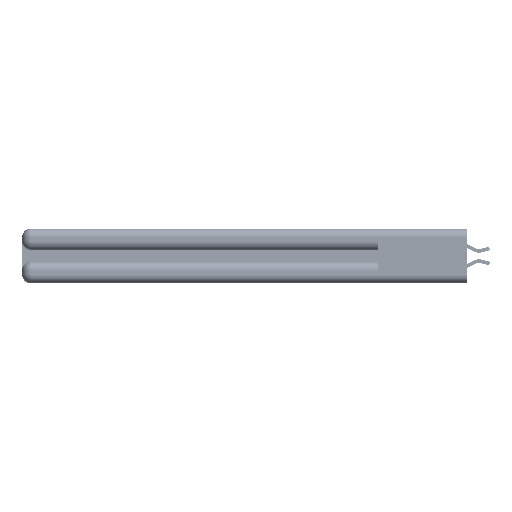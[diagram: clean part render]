
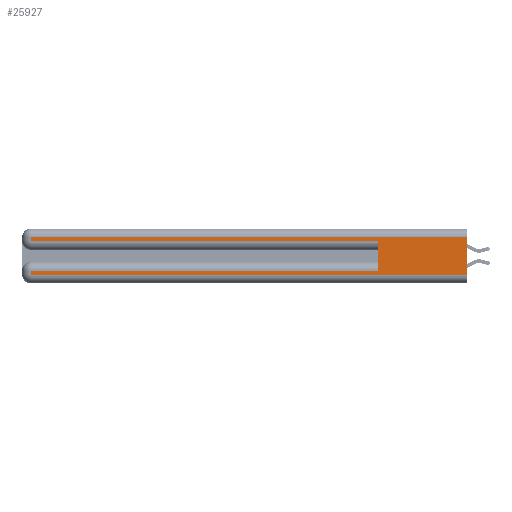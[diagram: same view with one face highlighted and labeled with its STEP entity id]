
A CAD part, left-side view. The second image highlights one B-rep face of the part: STEP entity #25927.
In plain terms, the highlighted planar face has unit normal (-1, 0, 0).
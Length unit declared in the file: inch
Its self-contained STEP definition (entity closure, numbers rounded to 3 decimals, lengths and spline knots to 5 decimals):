
#22 = CARTESIAN_POINT ( 'NONE',  ( 0., 0., 0.31 ) ) ;
#746 = VECTOR ( 'NONE', #11568, 39.37008 ) ;
#1099 = EDGE_CURVE ( 'NONE', #55158, #27219, #12413, .T. ) ;
#2362 = VECTOR ( 'NONE', #32102, 39.37008 ) ;
#2492 = CARTESIAN_POINT ( 'NONE',  ( 0., 2.94, 0.37 ) ) ;
#2868 = EDGE_CURVE ( 'NONE', #38556, #27219, #19186, .T. ) ;
#3260 = ORIENTED_EDGE ( 'NONE', *, *, #47919, .T. ) ;
#3585 = VERTEX_POINT ( 'NONE', #31854 ) ;
#3756 = ORIENTED_EDGE ( 'NONE', *, *, #12928, .F. ) ;
#5127 = CARTESIAN_POINT ( 'NONE',  ( 0., 0., 0.37 ) ) ;
#8975 = CARTESIAN_POINT ( 'NONE',  ( 0., 2.94, 0.37 ) ) ;
#9656 = PLANE ( 'NONE',  #36478 ) ;
#11568 = DIRECTION ( 'NONE',  ( 0., 0., -1. ) ) ;
#11847 = VERTEX_POINT ( 'NONE', #57214 ) ;
#12413 = LINE ( 'NONE', #34337, #36238 ) ;
#12446 = CARTESIAN_POINT ( 'NONE',  ( 0., 0., 0.31 ) ) ;
#12928 = EDGE_CURVE ( 'NONE', #46204, #11847, #29119, .T. ) ;
#14068 = CARTESIAN_POINT ( 'NONE',  ( 0., 0., 0.285 ) ) ;
#14163 = DIRECTION ( 'NONE',  ( 0., 0., -1. ) ) ;
#17338 = FACE_OUTER_BOUND ( 'NONE', #51139, .T. ) ;
#17996 = CARTESIAN_POINT ( 'NONE',  ( 0., 0., 0.085 ) ) ;
#18508 = DIRECTION ( 'NONE',  ( 1., 0., 0. ) ) ;
#19158 = EDGE_CURVE ( 'NONE', #28512, #11847, #53413, .T. ) ;
#19186 = LINE ( 'NONE', #36012, #53356 ) ;
#19574 = ORIENTED_EDGE ( 'NONE', *, *, #30008, .T. ) ;
#20158 = VECTOR ( 'NONE', #40652, 39.37008 ) ;
#20727 = EDGE_CURVE ( 'NONE', #3585, #38556, #24746, .T. ) ;
#22136 = LINE ( 'NONE', #17996, #44464 ) ;
#23123 = DIRECTION ( 'NONE',  ( 0., -1., 0. ) ) ;
#24746 = LINE ( 'NONE', #2492, #746 ) ;
#25570 = CARTESIAN_POINT ( 'NONE',  ( 0., 2.94, 0.285 ) ) ;
#25927 = ADVANCED_FACE ( 'NONE', ( #17338 ), #9656, .F. ) ;
#27219 = VERTEX_POINT ( 'NONE', #52904 ) ;
#27251 = DIRECTION ( 'NONE',  ( 0., -1., 0. ) ) ;
#28512 = VERTEX_POINT ( 'NONE', #25570 ) ;
#29119 = LINE ( 'NONE', #54239, #2362 ) ;
#30008 = EDGE_CURVE ( 'NONE', #55158, #52721, #32043, .T. ) ;
#31700 = DIRECTION ( 'NONE',  ( 0., 1., 0. ) ) ;
#31854 = CARTESIAN_POINT ( 'NONE',  ( 0., 2.94, 0.085 ) ) ;
#32043 = LINE ( 'NONE', #22, #20158 ) ;
#32102 = DIRECTION ( 'NONE',  ( 0., 0., 1. ) ) ;
#34337 = CARTESIAN_POINT ( 'NONE',  ( 0., 0., 0.37 ) ) ;
#34374 = CARTESIAN_POINT ( 'NONE',  ( 0., 2.94, 0.06 ) ) ;
#35749 = EDGE_CURVE ( 'NONE', #52721, #28512, #53698, .T. ) ;
#36012 = CARTESIAN_POINT ( 'NONE',  ( 0., 0., 0.06 ) ) ;
#36238 = VECTOR ( 'NONE', #52011, 39.37008 ) ;
#36478 = AXIS2_PLACEMENT_3D ( 'NONE', #5127, #18508, #14163 ) ;
#38556 = VERTEX_POINT ( 'NONE', #34374 ) ;
#40096 = ORIENTED_EDGE ( 'NONE', *, *, #35749, .T. ) ;
#40652 = DIRECTION ( 'NONE',  ( 0., 1., 0. ) ) ;
#41892 = VECTOR ( 'NONE', #44775, 39.37008 ) ;
#43265 = CARTESIAN_POINT ( 'NONE',  ( 0., 0.6, 0.085 ) ) ;
#43667 = ORIENTED_EDGE ( 'NONE', *, *, #20727, .T. ) ;
#44464 = VECTOR ( 'NONE', #31700, 39.37008 ) ;
#44775 = DIRECTION ( 'NONE',  ( 0., 0., -1. ) ) ;
#46204 = VERTEX_POINT ( 'NONE', #43265 ) ;
#47919 = EDGE_CURVE ( 'NONE', #46204, #3585, #22136, .T. ) ;
#51139 = EDGE_LOOP ( 'NONE', ( #57848, #19574, #40096, #51595, #3756, #3260, #43667, #57627 ) ) ;
#51595 = ORIENTED_EDGE ( 'NONE', *, *, #19158, .T. ) ;
#52011 = DIRECTION ( 'NONE',  ( 0., 0., -1. ) ) ;
#52024 = VECTOR ( 'NONE', #23123, 39.37008 ) ;
#52721 = VERTEX_POINT ( 'NONE', #55229 ) ;
#52904 = CARTESIAN_POINT ( 'NONE',  ( 0., 0., 0.06 ) ) ;
#53356 = VECTOR ( 'NONE', #27251, 39.37008 ) ;
#53413 = LINE ( 'NONE', #14068, #52024 ) ;
#53698 = LINE ( 'NONE', #8975, #41892 ) ;
#54239 = CARTESIAN_POINT ( 'NONE',  ( 0., 0.6, 0.145 ) ) ;
#55158 = VERTEX_POINT ( 'NONE', #12446 ) ;
#55229 = CARTESIAN_POINT ( 'NONE',  ( 0., 2.94, 0.31 ) ) ;
#57214 = CARTESIAN_POINT ( 'NONE',  ( 0., 0.6, 0.285 ) ) ;
#57627 = ORIENTED_EDGE ( 'NONE', *, *, #2868, .T. ) ;
#57848 = ORIENTED_EDGE ( 'NONE', *, *, #1099, .F. ) ;
